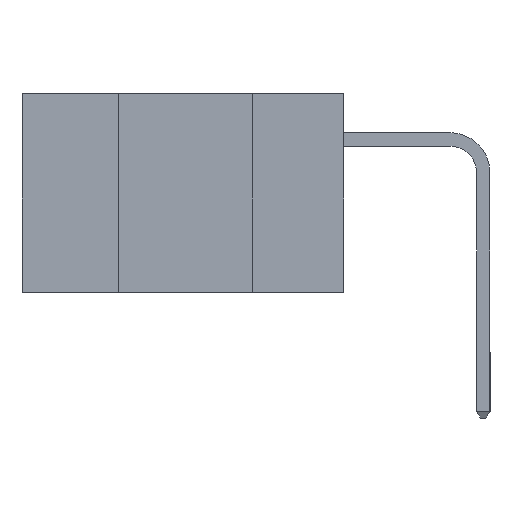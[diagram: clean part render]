
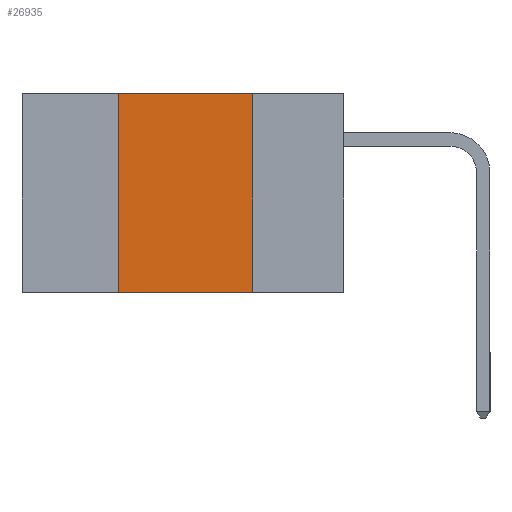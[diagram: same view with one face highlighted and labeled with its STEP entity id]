
A CAD part, left-side view. The second image highlights one B-rep face of the part: STEP entity #26935.
In plain terms, the highlighted planar face has unit normal (-1, 0, 0).
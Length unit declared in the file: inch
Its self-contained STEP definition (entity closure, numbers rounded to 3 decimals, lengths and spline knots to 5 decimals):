
#355 = CARTESIAN_POINT ( 'NONE',  ( 0., 0.42, 0. ) ) ;
#776 = PLANE ( 'NONE',  #1042 ) ;
#799 = LINE ( 'NONE', #2623, #25396 ) ;
#1042 = AXIS2_PLACEMENT_3D ( 'NONE', #5639, #22239, #8041 ) ;
#2556 = CARTESIAN_POINT ( 'NONE',  ( 0., 0.6, -0.37 ) ) ;
#2623 = CARTESIAN_POINT ( 'NONE',  ( 0., 0.17, 0. ) ) ;
#3317 = EDGE_CURVE ( 'NONE', #29765, #8664, #799, .T. ) ;
#3322 = CARTESIAN_POINT ( 'NONE',  ( 0., 0.6, 0. ) ) ;
#3839 = ORIENTED_EDGE ( 'NONE', *, *, #25233, .F. ) ;
#5639 = CARTESIAN_POINT ( 'NONE',  ( 0., 0.6, 0. ) ) ;
#8041 = DIRECTION ( 'NONE',  ( 0., 0., -1. ) ) ;
#8664 = VERTEX_POINT ( 'NONE', #17745 ) ;
#8735 = ORIENTED_EDGE ( 'NONE', *, *, #10225, .F. ) ;
#10225 = EDGE_CURVE ( 'NONE', #10728, #29765, #20173, .T. ) ;
#10728 = VERTEX_POINT ( 'NONE', #355 ) ;
#10823 = VECTOR ( 'NONE', #14493, 39.37008 ) ;
#11231 = LINE ( 'NONE', #13665, #16820 ) ;
#13149 = VECTOR ( 'NONE', #17658, 39.37008 ) ;
#13589 = ORIENTED_EDGE ( 'NONE', *, *, #3317, .F. ) ;
#13665 = CARTESIAN_POINT ( 'NONE',  ( 0., 0.42, 0. ) ) ;
#14493 = DIRECTION ( 'NONE',  ( 0., -1., 0. ) ) ;
#16820 = VECTOR ( 'NONE', #20773, 39.37008 ) ;
#17658 = DIRECTION ( 'NONE',  ( 0., -1., 0. ) ) ;
#17745 = CARTESIAN_POINT ( 'NONE',  ( 0., 0.17, -0.37 ) ) ;
#19167 = ORIENTED_EDGE ( 'NONE', *, *, #23655, .T. ) ;
#20173 = LINE ( 'NONE', #3322, #13149 ) ;
#20773 = DIRECTION ( 'NONE',  ( 0., 0., 1. ) ) ;
#22239 = DIRECTION ( 'NONE',  ( 1., 0., 0. ) ) ;
#22465 = VERTEX_POINT ( 'NONE', #26882 ) ;
#22950 = FACE_OUTER_BOUND ( 'NONE', #26762, .T. ) ;
#23655 = EDGE_CURVE ( 'NONE', #22465, #8664, #29667, .T. ) ;
#24051 = DIRECTION ( 'NONE',  ( 0., 0., -1. ) ) ;
#25233 = EDGE_CURVE ( 'NONE', #22465, #10728, #11231, .T. ) ;
#25396 = VECTOR ( 'NONE', #24051, 39.37008 ) ;
#26758 = CARTESIAN_POINT ( 'NONE',  ( 0., 0.17, 0. ) ) ;
#26762 = EDGE_LOOP ( 'NONE', ( #13589, #8735, #3839, #19167 ) ) ;
#26882 = CARTESIAN_POINT ( 'NONE',  ( 0., 0.42, -0.37 ) ) ;
#26935 = ADVANCED_FACE ( 'NONE', ( #22950 ), #776, .F. ) ;
#29667 = LINE ( 'NONE', #2556, #10823 ) ;
#29765 = VERTEX_POINT ( 'NONE', #26758 ) ;
